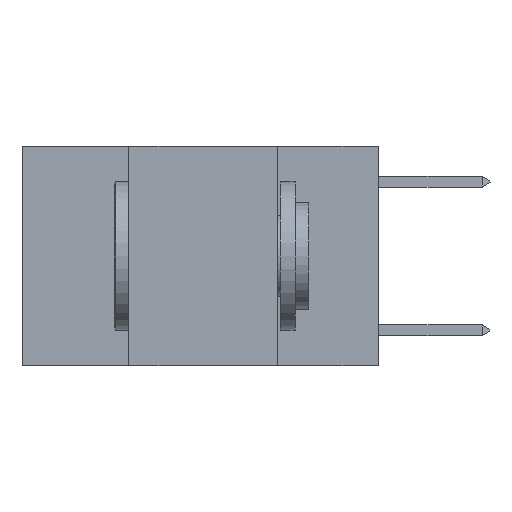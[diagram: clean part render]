
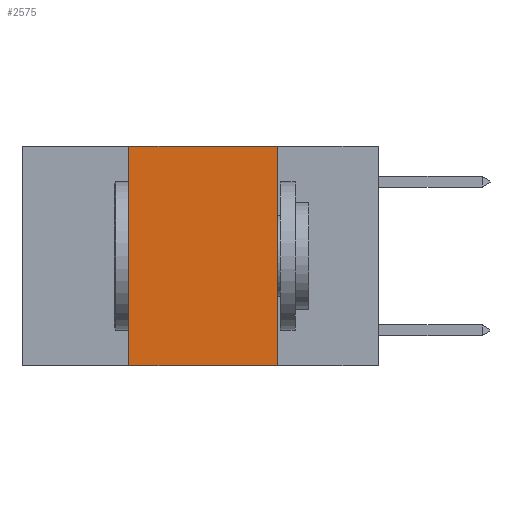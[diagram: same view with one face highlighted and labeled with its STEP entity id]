
A CAD part, left-side view. The second image highlights one B-rep face of the part: STEP entity #2575.
In plain terms, the highlighted planar face has unit normal (-1, 0, 0).
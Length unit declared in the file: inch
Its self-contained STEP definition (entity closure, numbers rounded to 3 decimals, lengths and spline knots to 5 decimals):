
#308 = ORIENTED_EDGE ( 'NONE', *, *, #416, .F. ) ;
#323 = ORIENTED_EDGE ( 'NONE', *, *, #6499, .F. ) ;
#416 = EDGE_CURVE ( 'NONE', #7307, #2454, #10310, .T. ) ;
#538 = VECTOR ( 'NONE', #6939, 39.37008 ) ;
#783 = AXIS2_PLACEMENT_3D ( 'NONE', #3294, #3266, #3237 ) ;
#1568 = CARTESIAN_POINT ( 'NONE',  ( 0., 0.17, -0.37 ) ) ;
#2386 = LINE ( 'NONE', #4237, #6781 ) ;
#2393 = ORIENTED_EDGE ( 'NONE', *, *, #3094, .T. ) ;
#2398 = FACE_OUTER_BOUND ( 'NONE', #5862, .T. ) ;
#2454 = VERTEX_POINT ( 'NONE', #5613 ) ;
#2575 = ADVANCED_FACE ( 'NONE', ( #2398 ), #3678, .F. ) ;
#2741 = CARTESIAN_POINT ( 'NONE',  ( 0., 0.6, 0. ) ) ;
#3094 = EDGE_CURVE ( 'NONE', #10247, #3675, #2386, .T. ) ;
#3237 = DIRECTION ( 'NONE',  ( 0., 0., -1. ) ) ;
#3266 = DIRECTION ( 'NONE',  ( 1., 0., 0. ) ) ;
#3294 = CARTESIAN_POINT ( 'NONE',  ( 0., 0.6, 0. ) ) ;
#3411 = ORIENTED_EDGE ( 'NONE', *, *, #8549, .F. ) ;
#3675 = VERTEX_POINT ( 'NONE', #1568 ) ;
#3678 = PLANE ( 'NONE',  #783 ) ;
#4237 = CARTESIAN_POINT ( 'NONE',  ( 0., 0.6, -0.37 ) ) ;
#5276 = CARTESIAN_POINT ( 'NONE',  ( 0., 0.42, 0. ) ) ;
#5613 = CARTESIAN_POINT ( 'NONE',  ( 0., 0.17, 0. ) ) ;
#5654 = DIRECTION ( 'NONE',  ( 0., -1., 0. ) ) ;
#5862 = EDGE_LOOP ( 'NONE', ( #3411, #308, #323, #2393 ) ) ;
#6140 = CARTESIAN_POINT ( 'NONE',  ( 0., 0.17, 0. ) ) ;
#6499 = EDGE_CURVE ( 'NONE', #10247, #7307, #9874, .T. ) ;
#6781 = VECTOR ( 'NONE', #7500, 39.37008 ) ;
#6908 = DIRECTION ( 'NONE',  ( 0., 0., 1. ) ) ;
#6939 = DIRECTION ( 'NONE',  ( 0., 0., -1. ) ) ;
#7094 = CARTESIAN_POINT ( 'NONE',  ( 0., 0.42, -0.37 ) ) ;
#7199 = LINE ( 'NONE', #6140, #538 ) ;
#7307 = VERTEX_POINT ( 'NONE', #10422 ) ;
#7500 = DIRECTION ( 'NONE',  ( 0., -1., 0. ) ) ;
#7732 = VECTOR ( 'NONE', #6908, 39.37008 ) ;
#8441 = VECTOR ( 'NONE', #5654, 39.37008 ) ;
#8549 = EDGE_CURVE ( 'NONE', #2454, #3675, #7199, .T. ) ;
#9874 = LINE ( 'NONE', #5276, #7732 ) ;
#10247 = VERTEX_POINT ( 'NONE', #7094 ) ;
#10310 = LINE ( 'NONE', #2741, #8441 ) ;
#10422 = CARTESIAN_POINT ( 'NONE',  ( 0., 0.42, 0. ) ) ;
